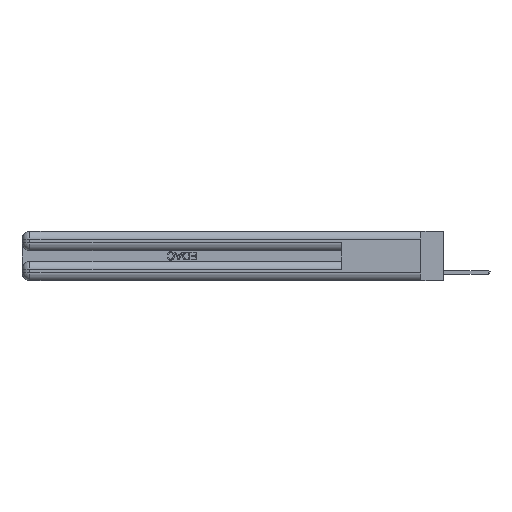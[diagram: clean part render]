
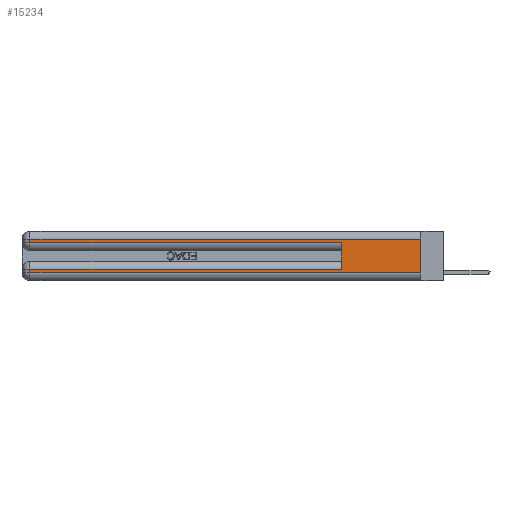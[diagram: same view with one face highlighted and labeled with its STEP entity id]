
A CAD part, left-side view. The second image highlights one B-rep face of the part: STEP entity #15234.
In plain terms, the highlighted planar face has unit normal (-1, 0, 0).
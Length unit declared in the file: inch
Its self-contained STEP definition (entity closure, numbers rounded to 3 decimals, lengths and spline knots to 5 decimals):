
#1155 = ORIENTED_EDGE ( 'NONE', *, *, #26185, .T. ) ;
#1156 = VERTEX_POINT ( 'NONE', #17143 ) ;
#1608 = LINE ( 'NONE', #27760, #13317 ) ;
#1958 = EDGE_CURVE ( 'NONE', #11589, #16942, #1608, .T. ) ;
#2282 = LINE ( 'NONE', #12724, #8508 ) ;
#2789 = VERTEX_POINT ( 'NONE', #27286 ) ;
#3372 = DIRECTION ( 'NONE',  ( 0., -1., 0. ) ) ;
#3527 = ORIENTED_EDGE ( 'NONE', *, *, #25167, .F. ) ;
#3582 = DIRECTION ( 'NONE',  ( 1., 0., 0. ) ) ;
#3821 = ORIENTED_EDGE ( 'NONE', *, *, #27444, .T. ) ;
#4583 = LINE ( 'NONE', #23213, #12745 ) ;
#4713 = CARTESIAN_POINT ( 'NONE',  ( 0., 0.6, 0.145 ) ) ;
#5985 = DIRECTION ( 'NONE',  ( 0., 0., -1. ) ) ;
#6026 = LINE ( 'NONE', #32169, #25585 ) ;
#6125 = ORIENTED_EDGE ( 'NONE', *, *, #30735, .F. ) ;
#6173 = EDGE_CURVE ( 'NONE', #18087, #12750, #31300, .T. ) ;
#7352 = EDGE_CURVE ( 'NONE', #12750, #2789, #14770, .T. ) ;
#7617 = VECTOR ( 'NONE', #31472, 39.37008 ) ;
#7648 = ORIENTED_EDGE ( 'NONE', *, *, #6173, .T. ) ;
#8404 = CARTESIAN_POINT ( 'NONE',  ( 0., 2.94, 0.06 ) ) ;
#8508 = VECTOR ( 'NONE', #29301, 39.37008 ) ;
#8551 = PLANE ( 'NONE',  #21971 ) ;
#8722 = CARTESIAN_POINT ( 'NONE',  ( 0., 0., 0.37 ) ) ;
#9330 = DIRECTION ( 'NONE',  ( 0., 0., 1. ) ) ;
#9565 = VERTEX_POINT ( 'NONE', #15532 ) ;
#10266 = VECTOR ( 'NONE', #9330, 39.37008 ) ;
#11170 = VECTOR ( 'NONE', #15903, 39.37008 ) ;
#11290 = FACE_OUTER_BOUND ( 'NONE', #31481, .T. ) ;
#11589 = VERTEX_POINT ( 'NONE', #31463 ) ;
#12274 = CARTESIAN_POINT ( 'NONE',  ( 0., 0.6, 0.085 ) ) ;
#12724 = CARTESIAN_POINT ( 'NONE',  ( 0., 0., 0.085 ) ) ;
#12745 = VECTOR ( 'NONE', #14850, 39.37008 ) ;
#12750 = VERTEX_POINT ( 'NONE', #8404 ) ;
#13317 = VECTOR ( 'NONE', #3372, 39.37008 ) ;
#14641 = LINE ( 'NONE', #4713, #10266 ) ;
#14770 = LINE ( 'NONE', #22789, #24407 ) ;
#14850 = DIRECTION ( 'NONE',  ( 0., 0., -1. ) ) ;
#15234 = ADVANCED_FACE ( 'NONE', ( #11290 ), #8551, .F. ) ;
#15532 = CARTESIAN_POINT ( 'NONE',  ( 0., 0., 0.31 ) ) ;
#15903 = DIRECTION ( 'NONE',  ( 0., 0., -1. ) ) ;
#16561 = CARTESIAN_POINT ( 'NONE',  ( 0., 0.6, 0.285 ) ) ;
#16942 = VERTEX_POINT ( 'NONE', #16561 ) ;
#17143 = CARTESIAN_POINT ( 'NONE',  ( 0., 2.94, 0.31 ) ) ;
#18087 = VERTEX_POINT ( 'NONE', #25489 ) ;
#21743 = VERTEX_POINT ( 'NONE', #12274 ) ;
#21971 = AXIS2_PLACEMENT_3D ( 'NONE', #8722, #3582, #5985 ) ;
#22452 = DIRECTION ( 'NONE',  ( 0., -1., 0. ) ) ;
#22789 = CARTESIAN_POINT ( 'NONE',  ( 0., 0., 0.06 ) ) ;
#23213 = CARTESIAN_POINT ( 'NONE',  ( 0., 0., 0.37 ) ) ;
#23863 = ORIENTED_EDGE ( 'NONE', *, *, #7352, .T. ) ;
#24261 = LINE ( 'NONE', #26995, #11170 ) ;
#24407 = VECTOR ( 'NONE', #22452, 39.37008 ) ;
#25167 = EDGE_CURVE ( 'NONE', #9565, #2789, #4583, .T. ) ;
#25489 = CARTESIAN_POINT ( 'NONE',  ( 0., 2.94, 0.085 ) ) ;
#25585 = VECTOR ( 'NONE', #26867, 39.37008 ) ;
#26185 = EDGE_CURVE ( 'NONE', #1156, #11589, #24261, .T. ) ;
#26867 = DIRECTION ( 'NONE',  ( 0., 1., 0. ) ) ;
#26995 = CARTESIAN_POINT ( 'NONE',  ( 0., 2.94, 0.37 ) ) ;
#27286 = CARTESIAN_POINT ( 'NONE',  ( 0., 0., 0.06 ) ) ;
#27444 = EDGE_CURVE ( 'NONE', #21743, #18087, #2282, .T. ) ;
#27760 = CARTESIAN_POINT ( 'NONE',  ( 0., 0., 0.285 ) ) ;
#28745 = CARTESIAN_POINT ( 'NONE',  ( 0., 2.94, 0.37 ) ) ;
#29301 = DIRECTION ( 'NONE',  ( 0., 1., 0. ) ) ;
#30735 = EDGE_CURVE ( 'NONE', #21743, #16942, #14641, .T. ) ;
#31300 = LINE ( 'NONE', #28745, #7617 ) ;
#31406 = ORIENTED_EDGE ( 'NONE', *, *, #32739, .T. ) ;
#31463 = CARTESIAN_POINT ( 'NONE',  ( 0., 2.94, 0.285 ) ) ;
#31472 = DIRECTION ( 'NONE',  ( 0., 0., -1. ) ) ;
#31481 = EDGE_LOOP ( 'NONE', ( #3527, #31406, #1155, #33606, #6125, #3821, #7648, #23863 ) ) ;
#32169 = CARTESIAN_POINT ( 'NONE',  ( 0., 0., 0.31 ) ) ;
#32739 = EDGE_CURVE ( 'NONE', #9565, #1156, #6026, .T. ) ;
#33606 = ORIENTED_EDGE ( 'NONE', *, *, #1958, .T. ) ;
